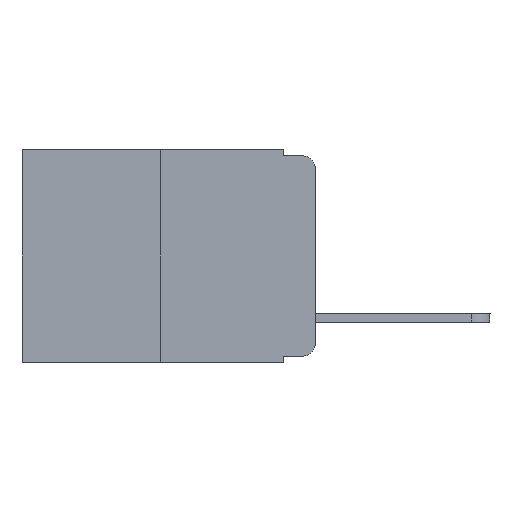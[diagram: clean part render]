
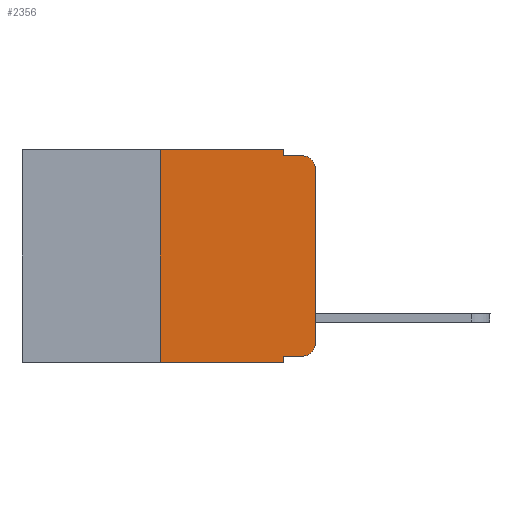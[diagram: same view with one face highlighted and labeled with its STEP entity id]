
A CAD part, left-side view. The second image highlights one B-rep face of the part: STEP entity #2356.
In plain terms, the highlighted planar face has unit normal (-1, 0, 0).
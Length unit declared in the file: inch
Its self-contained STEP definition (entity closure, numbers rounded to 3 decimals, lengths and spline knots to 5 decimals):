
#242 = VECTOR ( 'NONE', #7154, 39.37008 ) ;
#256 = EDGE_CURVE ( 'NONE', #20030, #15982, #21647, .T. ) ;
#330 = CARTESIAN_POINT ( 'NONE',  ( 0., 0., 0. ) ) ;
#644 = ORIENTED_EDGE ( 'NONE', *, *, #256, .F. ) ;
#655 = EDGE_CURVE ( 'NONE', #1987, #17365, #11264, .T. ) ;
#1597 = DIRECTION ( 'NONE',  ( 0., 0., -1. ) ) ;
#1654 = EDGE_CURVE ( 'NONE', #12933, #20030, #4751, .T. ) ;
#1811 = DIRECTION ( 'NONE',  ( 0., 0., -1. ) ) ;
#1987 = VERTEX_POINT ( 'NONE', #17964 ) ;
#2088 = AXIS2_PLACEMENT_3D ( 'NONE', #3253, #18737, #1597 ) ;
#2105 = ORIENTED_EDGE ( 'NONE', *, *, #13730, .F. ) ;
#2356 = ADVANCED_FACE ( 'NONE', ( #13831 ), #17061, .F. ) ;
#2602 = CARTESIAN_POINT ( 'NONE',  ( 0., 0.051, -0.343 ) ) ;
#2645 = LINE ( 'NONE', #7681, #12821 ) ;
#2756 = ORIENTED_EDGE ( 'NONE', *, *, #6394, .T. ) ;
#2870 = ORIENTED_EDGE ( 'NONE', *, *, #18834, .F. ) ;
#3253 = CARTESIAN_POINT ( 'NONE',  ( 0., 0.02, -0.313 ) ) ;
#3275 = CARTESIAN_POINT ( 'NONE',  ( 0., 0.02, -0.01 ) ) ;
#3438 = CARTESIAN_POINT ( 'NONE',  ( 0., 0.25, -0.343 ) ) ;
#3511 = LINE ( 'NONE', #17102, #16010 ) ;
#3533 = EDGE_CURVE ( 'NONE', #17365, #15294, #13467, .T. ) ;
#4012 = VERTEX_POINT ( 'NONE', #7384 ) ;
#4253 = DIRECTION ( 'NONE',  ( 0., 0., -1. ) ) ;
#4751 = LINE ( 'NONE', #17085, #6924 ) ;
#4856 = DIRECTION ( 'NONE',  ( 0., 0., 1. ) ) ;
#6143 = DIRECTION ( 'NONE',  ( -1., 0., 0. ) ) ;
#6196 = VERTEX_POINT ( 'NONE', #3438 ) ;
#6394 = EDGE_CURVE ( 'NONE', #6196, #10384, #2645, .T. ) ;
#6746 = VECTOR ( 'NONE', #7730, 39.37008 ) ;
#6924 = VECTOR ( 'NONE', #20113, 39.37008 ) ;
#7043 = CARTESIAN_POINT ( 'NONE',  ( 0., 0., -0.313 ) ) ;
#7149 = AXIS2_PLACEMENT_3D ( 'NONE', #7782, #6143, #12884 ) ;
#7154 = DIRECTION ( 'NONE',  ( 0., 0., 1. ) ) ;
#7384 = CARTESIAN_POINT ( 'NONE',  ( 0., 0., -0.03 ) ) ;
#7681 = CARTESIAN_POINT ( 'NONE',  ( 0., 0.473, -0.343 ) ) ;
#7730 = DIRECTION ( 'NONE',  ( 0., -1., 0. ) ) ;
#7782 = CARTESIAN_POINT ( 'NONE',  ( 0., 0.02, -0.03 ) ) ;
#9063 = CARTESIAN_POINT ( 'NONE',  ( 0., 0.473, 0. ) ) ;
#9171 = CARTESIAN_POINT ( 'NONE',  ( 0., 0.25, 0. ) ) ;
#9452 = AXIS2_PLACEMENT_3D ( 'NONE', #9063, #20628, #1811 ) ;
#9473 = ORIENTED_EDGE ( 'NONE', *, *, #1654, .F. ) ;
#9516 = CARTESIAN_POINT ( 'NONE',  ( 0., 0.051, -0.01 ) ) ;
#10163 = ORIENTED_EDGE ( 'NONE', *, *, #18703, .T. ) ;
#10384 = VERTEX_POINT ( 'NONE', #2602 ) ;
#10949 = LINE ( 'NONE', #21625, #12267 ) ;
#11128 = DIRECTION ( 'NONE',  ( 0., -1., 0. ) ) ;
#11264 = LINE ( 'NONE', #16371, #17355 ) ;
#11931 = EDGE_CURVE ( 'NONE', #6196, #14930, #15180, .T. ) ;
#11998 = DIRECTION ( 'NONE',  ( 0., -1., 0. ) ) ;
#12251 = LINE ( 'NONE', #330, #242 ) ;
#12267 = VECTOR ( 'NONE', #4253, 39.37008 ) ;
#12347 = CARTESIAN_POINT ( 'NONE',  ( 0., 0.02, -0.333 ) ) ;
#12803 = DIRECTION ( 'NONE',  ( 0., -1., 0. ) ) ;
#12821 = VECTOR ( 'NONE', #11128, 39.37008 ) ;
#12884 = DIRECTION ( 'NONE',  ( 0., 0., -1. ) ) ;
#12933 = VERTEX_POINT ( 'NONE', #19215 ) ;
#13467 = CIRCLE ( 'NONE', #2088, 0.02 ) ;
#13730 = EDGE_CURVE ( 'NONE', #1987, #10384, #10949, .T. ) ;
#13831 = FACE_OUTER_BOUND ( 'NONE', #17993, .T. ) ;
#14046 = VECTOR ( 'NONE', #4856, 39.37008 ) ;
#14930 = VERTEX_POINT ( 'NONE', #9171 ) ;
#15180 = LINE ( 'NONE', #18311, #14046 ) ;
#15294 = VERTEX_POINT ( 'NONE', #7043 ) ;
#15361 = EDGE_CURVE ( 'NONE', #15294, #4012, #12251, .T. ) ;
#15982 = VERTEX_POINT ( 'NONE', #3275 ) ;
#16010 = VECTOR ( 'NONE', #11998, 39.37008 ) ;
#16348 = CIRCLE ( 'NONE', #7149, 0.02 ) ;
#16371 = CARTESIAN_POINT ( 'NONE',  ( 0., 0.051, -0.333 ) ) ;
#16810 = ORIENTED_EDGE ( 'NONE', *, *, #11931, .F. ) ;
#16897 = CARTESIAN_POINT ( 'NONE',  ( 0., 0.051, -0.01 ) ) ;
#17061 = PLANE ( 'NONE',  #9452 ) ;
#17085 = CARTESIAN_POINT ( 'NONE',  ( 0., 0.051, 0. ) ) ;
#17102 = CARTESIAN_POINT ( 'NONE',  ( 0., 0.473, 0. ) ) ;
#17355 = VECTOR ( 'NONE', #12803, 39.37008 ) ;
#17365 = VERTEX_POINT ( 'NONE', #12347 ) ;
#17964 = CARTESIAN_POINT ( 'NONE',  ( 0., 0.051, -0.333 ) ) ;
#17993 = EDGE_LOOP ( 'NONE', ( #21816, #10163, #644, #9473, #2870, #16810, #2756, #2105, #20816, #19829 ) ) ;
#18311 = CARTESIAN_POINT ( 'NONE',  ( 0., 0.25, 0. ) ) ;
#18703 = EDGE_CURVE ( 'NONE', #4012, #15982, #16348, .T. ) ;
#18737 = DIRECTION ( 'NONE',  ( -1., 0., 0. ) ) ;
#18834 = EDGE_CURVE ( 'NONE', #14930, #12933, #3511, .T. ) ;
#19215 = CARTESIAN_POINT ( 'NONE',  ( 0., 0.051, 0. ) ) ;
#19829 = ORIENTED_EDGE ( 'NONE', *, *, #3533, .T. ) ;
#20030 = VERTEX_POINT ( 'NONE', #16897 ) ;
#20113 = DIRECTION ( 'NONE',  ( 0., 0., -1. ) ) ;
#20628 = DIRECTION ( 'NONE',  ( 1., 0., 0. ) ) ;
#20816 = ORIENTED_EDGE ( 'NONE', *, *, #655, .T. ) ;
#21625 = CARTESIAN_POINT ( 'NONE',  ( 0., 0.051, 0. ) ) ;
#21647 = LINE ( 'NONE', #9516, #6746 ) ;
#21816 = ORIENTED_EDGE ( 'NONE', *, *, #15361, .T. ) ;
